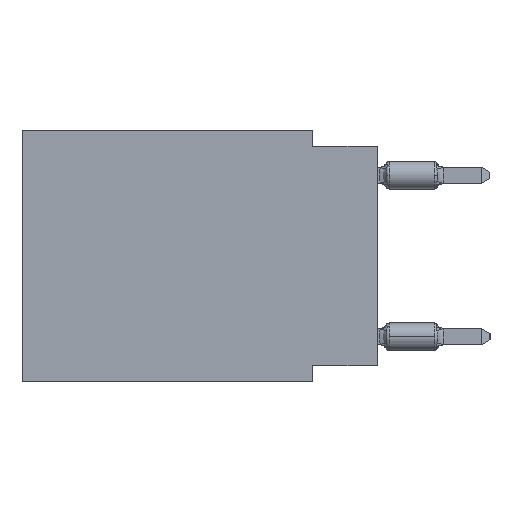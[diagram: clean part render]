
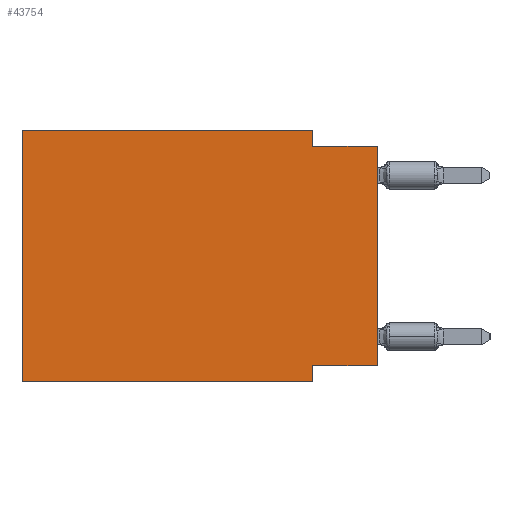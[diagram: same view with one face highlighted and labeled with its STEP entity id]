
A CAD part, left-side view. The second image highlights one B-rep face of the part: STEP entity #43754.
In plain terms, the highlighted planar face has unit normal (-1, 0, 0).
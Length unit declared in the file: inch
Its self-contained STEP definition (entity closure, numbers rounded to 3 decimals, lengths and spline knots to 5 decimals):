
#949 = CARTESIAN_POINT ( 'NONE',  ( 0., 0., -0.025 ) ) ;
#1005 = VERTEX_POINT ( 'NONE', #20719 ) ;
#1514 = DIRECTION ( 'NONE',  ( 1., 0., 0. ) ) ;
#2100 = CARTESIAN_POINT ( 'NONE',  ( 0., 0.1, -0.025 ) ) ;
#6678 = LINE ( 'NONE', #24993, #31968 ) ;
#6840 = ORIENTED_EDGE ( 'NONE', *, *, #39946, .F. ) ;
#6941 = DIRECTION ( 'NONE',  ( 0., -1., 0. ) ) ;
#8077 = ORIENTED_EDGE ( 'NONE', *, *, #13496, .F. ) ;
#9604 = LINE ( 'NONE', #31317, #40500 ) ;
#11156 = PLANE ( 'NONE',  #59224 ) ;
#11183 = DIRECTION ( 'NONE',  ( 0., -1., 0. ) ) ;
#12170 = ORIENTED_EDGE ( 'NONE', *, *, #59419, .F. ) ;
#12454 = VERTEX_POINT ( 'NONE', #16076 ) ;
#12995 = EDGE_CURVE ( 'NONE', #12454, #50975, #9604, .T. ) ;
#13063 = CARTESIAN_POINT ( 'NONE',  ( 0., 0., 0. ) ) ;
#13496 = EDGE_CURVE ( 'NONE', #23978, #28751, #51449, .T. ) ;
#14203 = LINE ( 'NONE', #24471, #46379 ) ;
#16076 = CARTESIAN_POINT ( 'NONE',  ( 0., 0.1, 0. ) ) ;
#17174 = ORIENTED_EDGE ( 'NONE', *, *, #12995, .F. ) ;
#18064 = DIRECTION ( 'NONE',  ( 0., 1., 0. ) ) ;
#18110 = ORIENTED_EDGE ( 'NONE', *, *, #21780, .F. ) ;
#18214 = CARTESIAN_POINT ( 'NONE',  ( 0., 0.55, 0. ) ) ;
#19902 = LINE ( 'NONE', #949, #39587 ) ;
#20719 = CARTESIAN_POINT ( 'NONE',  ( 0., 0., -0.025 ) ) ;
#21780 = EDGE_CURVE ( 'NONE', #28751, #37698, #14203, .T. ) ;
#23978 = VERTEX_POINT ( 'NONE', #54242 ) ;
#24471 = CARTESIAN_POINT ( 'NONE',  ( 0., 0.1, -0.39 ) ) ;
#24993 = CARTESIAN_POINT ( 'NONE',  ( 0., 0.55, -0.39 ) ) ;
#25516 = VECTOR ( 'NONE', #45387, 39.37008 ) ;
#26553 = LINE ( 'NONE', #13063, #37526 ) ;
#26827 = VERTEX_POINT ( 'NONE', #33848 ) ;
#27689 = CARTESIAN_POINT ( 'NONE',  ( 0., 0., -0.365 ) ) ;
#28751 = VERTEX_POINT ( 'NONE', #58787 ) ;
#31317 = CARTESIAN_POINT ( 'NONE',  ( 0., 0.1, 0. ) ) ;
#31324 = CARTESIAN_POINT ( 'NONE',  ( 0., 0.55, 0. ) ) ;
#31968 = VECTOR ( 'NONE', #11183, 39.37008 ) ;
#33848 = CARTESIAN_POINT ( 'NONE',  ( 0., 0.55, -0.39 ) ) ;
#35152 = EDGE_CURVE ( 'NONE', #26827, #57872, #35779, .T. ) ;
#35779 = LINE ( 'NONE', #40913, #25516 ) ;
#36133 = ORIENTED_EDGE ( 'NONE', *, *, #35152, .F. ) ;
#37526 = VECTOR ( 'NONE', #47370, 39.37008 ) ;
#37698 = VERTEX_POINT ( 'NONE', #56083 ) ;
#39587 = VECTOR ( 'NONE', #49431, 39.37008 ) ;
#39946 = EDGE_CURVE ( 'NONE', #50975, #1005, #19902, .T. ) ;
#40040 = EDGE_CURVE ( 'NONE', #23978, #1005, #26553, .T. ) ;
#40500 = VECTOR ( 'NONE', #54759, 39.37008 ) ;
#40913 = CARTESIAN_POINT ( 'NONE',  ( 0., 0.55, 0. ) ) ;
#40953 = LINE ( 'NONE', #31324, #42793 ) ;
#41925 = ORIENTED_EDGE ( 'NONE', *, *, #50415, .T. ) ;
#42793 = VECTOR ( 'NONE', #6941, 39.37008 ) ;
#43754 = ADVANCED_FACE ( 'NONE', ( #45467 ), #11156, .F. ) ;
#45387 = DIRECTION ( 'NONE',  ( 0., 0., 1. ) ) ;
#45467 = FACE_OUTER_BOUND ( 'NONE', #52843, .T. ) ;
#46379 = VECTOR ( 'NONE', #53668, 39.37008 ) ;
#47370 = DIRECTION ( 'NONE',  ( 0., 0., 1. ) ) ;
#48111 = ORIENTED_EDGE ( 'NONE', *, *, #40040, .T. ) ;
#49431 = DIRECTION ( 'NONE',  ( 0., -1., 0. ) ) ;
#50303 = CARTESIAN_POINT ( 'NONE',  ( 0., 0.55, 0. ) ) ;
#50415 = EDGE_CURVE ( 'NONE', #26827, #37698, #6678, .T. ) ;
#50975 = VERTEX_POINT ( 'NONE', #2100 ) ;
#51449 = LINE ( 'NONE', #27689, #61017 ) ;
#52843 = EDGE_LOOP ( 'NONE', ( #48111, #6840, #17174, #12170, #36133, #41925, #18110, #8077 ) ) ;
#53668 = DIRECTION ( 'NONE',  ( 0., 0., -1. ) ) ;
#54242 = CARTESIAN_POINT ( 'NONE',  ( 0., 0., -0.365 ) ) ;
#54759 = DIRECTION ( 'NONE',  ( 0., 0., -1. ) ) ;
#56083 = CARTESIAN_POINT ( 'NONE',  ( 0., 0.1, -0.39 ) ) ;
#57872 = VERTEX_POINT ( 'NONE', #18214 ) ;
#58787 = CARTESIAN_POINT ( 'NONE',  ( 0., 0.1, -0.365 ) ) ;
#59224 = AXIS2_PLACEMENT_3D ( 'NONE', #50303, #1514, #61110 ) ;
#59419 = EDGE_CURVE ( 'NONE', #57872, #12454, #40953, .T. ) ;
#61017 = VECTOR ( 'NONE', #18064, 39.37008 ) ;
#61110 = DIRECTION ( 'NONE',  ( 0., 0., -1. ) ) ;
